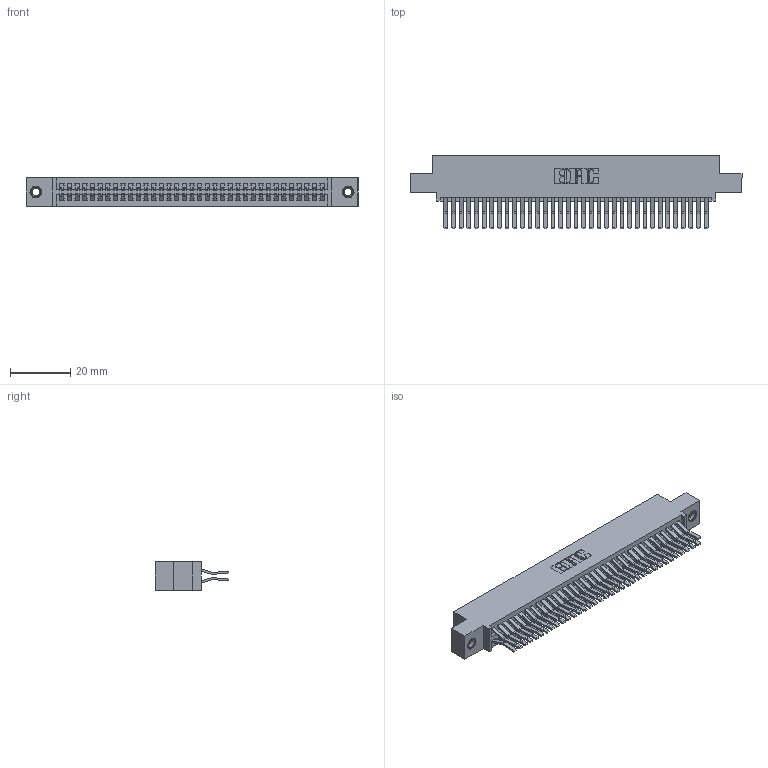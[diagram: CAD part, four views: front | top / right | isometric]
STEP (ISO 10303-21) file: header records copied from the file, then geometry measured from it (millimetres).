
FILE_DESCRIPTION (( 'STEP AP203' ), '1' );
FILE_NAME ('395-070-560-507.STEP', '2019-10-24T11:25:53', ( '' ), ( '' ), 'SwSTEP 2.0', 'SolidWorks 2016', '' );
FILE_SCHEMA (( 'CONFIG_CONTROL_DESIGN' ));
Length unit declared in the file: inch
Products named in the file (4): 345 Part_0.110 Offset - 0.156 Dia-TI; 345-292-001_560 Tail; 345-250-001_345-250-005-103; 395-070-560-507
Assembly tree (73 placements, depth 2):
  395-070-560-507
    345 Part_0.110 Offset - 0.156 Dia-TI
    345-292-001_560 Tail  x70
    345-250-001_345-250-005-103  x2
Bounding box: 110.11 x 24.45 x 9.4 mm (x, y, z)
Volume: 11003.1 mm3; surface area: 17429.6 mm2
Topology: 73 solids, 73 shells, 3830 faces, 11339 edges, 7458 vertices
Faces by surface type: plane 2426, cylinder 1388, cone 12, torus 4
Entity records: 29810 total; most frequent: CARTESIAN_POINT 4987, ORIENTED_EDGE 4914, DIRECTION 4435, EDGE_CURVE 2457, VECTOR 2161, LINE 2161, VERTEX_POINT 1632, AXIS2_PLACEMENT_3D 1137
